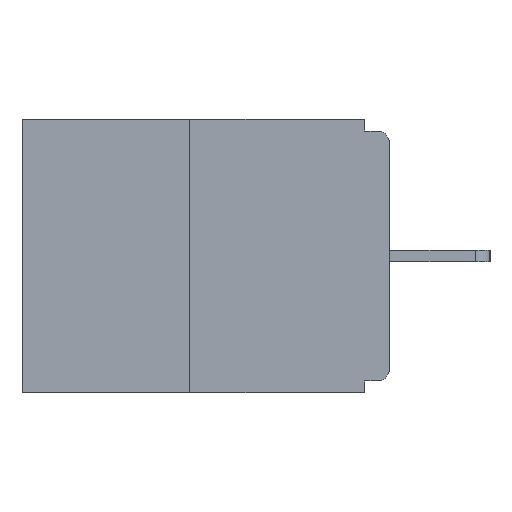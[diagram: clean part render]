
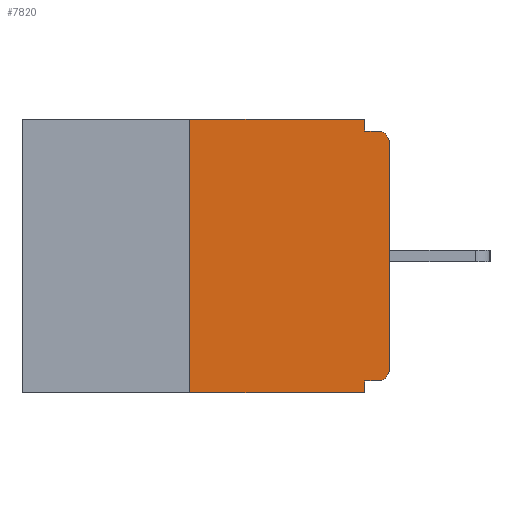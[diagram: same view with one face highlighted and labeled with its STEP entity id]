
A CAD part, left-side view. The second image highlights one B-rep face of the part: STEP entity #7820.
In plain terms, the highlighted planar face has unit normal (-1, 0, 0).
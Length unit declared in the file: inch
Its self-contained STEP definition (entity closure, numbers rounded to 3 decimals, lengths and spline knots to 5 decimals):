
#107 = DIRECTION ( 'NONE',  ( 0., 0., -1. ) ) ;
#194 = CARTESIAN_POINT ( 'NONE',  ( 0., 0.031, -0.015 ) ) ;
#774 = VERTEX_POINT ( 'NONE', #20372 ) ;
#1068 = CARTESIAN_POINT ( 'NONE',  ( 0., 0.015, -0.313 ) ) ;
#1338 = CARTESIAN_POINT ( 'NONE',  ( 0., 0.031, -0.343 ) ) ;
#1649 = CARTESIAN_POINT ( 'NONE',  ( 0., 0.031, -0.343 ) ) ;
#1908 = LINE ( 'NONE', #23898, #20549 ) ;
#2915 = LINE ( 'NONE', #9059, #10678 ) ;
#3018 = EDGE_CURVE ( 'NONE', #19893, #18446, #19276, .T. ) ;
#3280 = FACE_OUTER_BOUND ( 'NONE', #11662, .T. ) ;
#3738 = VERTEX_POINT ( 'NONE', #22603 ) ;
#3855 = DIRECTION ( 'NONE',  ( 0., 0., 1. ) ) ;
#3946 = AXIS2_PLACEMENT_3D ( 'NONE', #1068, #9276, #17248 ) ;
#4081 = VECTOR ( 'NONE', #10979, 39.37008 ) ;
#4439 = CARTESIAN_POINT ( 'NONE',  ( 0., 0.015, -0.03 ) ) ;
#4445 = ORIENTED_EDGE ( 'NONE', *, *, #15441, .F. ) ;
#5253 = CARTESIAN_POINT ( 'NONE',  ( 0., 0., 0. ) ) ;
#5824 = VECTOR ( 'NONE', #15744, 39.37008 ) ;
#6378 = DIRECTION ( 'NONE',  ( 0., 0., -1. ) ) ;
#7626 = CARTESIAN_POINT ( 'NONE',  ( 0., 0., -0.328 ) ) ;
#7820 = ADVANCED_FACE ( 'NONE', ( #3280 ), #11232, .F. ) ;
#8363 = VECTOR ( 'NONE', #13134, 39.37008 ) ;
#8448 = VERTEX_POINT ( 'NONE', #21889 ) ;
#8752 = EDGE_CURVE ( 'NONE', #8448, #23775, #13078, .T. ) ;
#9059 = CARTESIAN_POINT ( 'NONE',  ( 0., 0.031, 0. ) ) ;
#9276 = DIRECTION ( 'NONE',  ( -1., 0., 0. ) ) ;
#9626 = ORIENTED_EDGE ( 'NONE', *, *, #8752, .T. ) ;
#9677 = EDGE_CURVE ( 'NONE', #23457, #3738, #11603, .T. ) ;
#9801 = CIRCLE ( 'NONE', #20691, 0.015 ) ;
#9917 = ORIENTED_EDGE ( 'NONE', *, *, #3018, .T. ) ;
#10007 = EDGE_CURVE ( 'NONE', #19893, #24712, #1908, .T. ) ;
#10560 = ORIENTED_EDGE ( 'NONE', *, *, #19268, .F. ) ;
#10607 = CIRCLE ( 'NONE', #3946, 0.015 ) ;
#10678 = VECTOR ( 'NONE', #13244, 39.37008 ) ;
#10979 = DIRECTION ( 'NONE',  ( 0., 0., 1. ) ) ;
#11232 = PLANE ( 'NONE',  #19928 ) ;
#11281 = LINE ( 'NONE', #12868, #19151 ) ;
#11421 = ORIENTED_EDGE ( 'NONE', *, *, #12756, .T. ) ;
#11554 = LINE ( 'NONE', #1649, #8363 ) ;
#11603 = LINE ( 'NONE', #15906, #16869 ) ;
#11662 = EDGE_LOOP ( 'NONE', ( #20540, #25510, #9917, #10560, #18119, #11421, #9626, #19878, #13581, #4445 ) ) ;
#11789 = CARTESIAN_POINT ( 'NONE',  ( 0., 0.015, -0.328 ) ) ;
#12123 = VERTEX_POINT ( 'NONE', #13935 ) ;
#12756 = EDGE_CURVE ( 'NONE', #19973, #8448, #10607, .T. ) ;
#12868 = CARTESIAN_POINT ( 'NONE',  ( 0., 0.46, 0. ) ) ;
#13047 = EDGE_CURVE ( 'NONE', #23775, #3738, #9801, .T. ) ;
#13078 = LINE ( 'NONE', #5253, #4081 ) ;
#13123 = DIRECTION ( 'NONE',  ( 0., -1., 0. ) ) ;
#13134 = DIRECTION ( 'NONE',  ( 0., 0., -1. ) ) ;
#13244 = DIRECTION ( 'NONE',  ( 0., 0., -1. ) ) ;
#13581 = ORIENTED_EDGE ( 'NONE', *, *, #9677, .F. ) ;
#13935 = CARTESIAN_POINT ( 'NONE',  ( 0., 0.031, 0. ) ) ;
#14230 = DIRECTION ( 'NONE',  ( -1., 0., 0. ) ) ;
#15353 = CARTESIAN_POINT ( 'NONE',  ( 0., 0.46, -0.343 ) ) ;
#15441 = EDGE_CURVE ( 'NONE', #12123, #23457, #2915, .T. ) ;
#15479 = DIRECTION ( 'NONE',  ( 0., -1., 0. ) ) ;
#15622 = EDGE_CURVE ( 'NONE', #24712, #12123, #11281, .T. ) ;
#15744 = DIRECTION ( 'NONE',  ( 0., 1., 0. ) ) ;
#15906 = CARTESIAN_POINT ( 'NONE',  ( 0., 0., -0.015 ) ) ;
#16072 = VECTOR ( 'NONE', #13123, 39.37008 ) ;
#16869 = VECTOR ( 'NONE', #17615, 39.37008 ) ;
#17248 = DIRECTION ( 'NONE',  ( 0., 0., -1. ) ) ;
#17615 = DIRECTION ( 'NONE',  ( 0., -1., 0. ) ) ;
#17785 = DIRECTION ( 'NONE',  ( 1., 0., 0. ) ) ;
#18027 = EDGE_CURVE ( 'NONE', #19973, #774, #20049, .T. ) ;
#18119 = ORIENTED_EDGE ( 'NONE', *, *, #18027, .F. ) ;
#18446 = VERTEX_POINT ( 'NONE', #1338 ) ;
#19151 = VECTOR ( 'NONE', #15479, 39.37008 ) ;
#19268 = EDGE_CURVE ( 'NONE', #774, #18446, #11554, .T. ) ;
#19276 = LINE ( 'NONE', #15353, #16072 ) ;
#19414 = CARTESIAN_POINT ( 'NONE',  ( 0., 0., -0.03 ) ) ;
#19878 = ORIENTED_EDGE ( 'NONE', *, *, #13047, .T. ) ;
#19893 = VERTEX_POINT ( 'NONE', #21260 ) ;
#19928 = AXIS2_PLACEMENT_3D ( 'NONE', #25807, #17785, #107 ) ;
#19973 = VERTEX_POINT ( 'NONE', #11789 ) ;
#20049 = LINE ( 'NONE', #7626, #5824 ) ;
#20372 = CARTESIAN_POINT ( 'NONE',  ( 0., 0.031, -0.328 ) ) ;
#20540 = ORIENTED_EDGE ( 'NONE', *, *, #15622, .F. ) ;
#20549 = VECTOR ( 'NONE', #3855, 39.37008 ) ;
#20691 = AXIS2_PLACEMENT_3D ( 'NONE', #4439, #14230, #6378 ) ;
#21260 = CARTESIAN_POINT ( 'NONE',  ( 0., 0.25, -0.343 ) ) ;
#21889 = CARTESIAN_POINT ( 'NONE',  ( 0., 0., -0.313 ) ) ;
#22603 = CARTESIAN_POINT ( 'NONE',  ( 0., 0.015, -0.015 ) ) ;
#23445 = CARTESIAN_POINT ( 'NONE',  ( 0., 0.25, 0. ) ) ;
#23457 = VERTEX_POINT ( 'NONE', #194 ) ;
#23775 = VERTEX_POINT ( 'NONE', #19414 ) ;
#23898 = CARTESIAN_POINT ( 'NONE',  ( 0., 0.25, 0. ) ) ;
#24712 = VERTEX_POINT ( 'NONE', #23445 ) ;
#25510 = ORIENTED_EDGE ( 'NONE', *, *, #10007, .F. ) ;
#25807 = CARTESIAN_POINT ( 'NONE',  ( 0., 0.46, 0. ) ) ;
